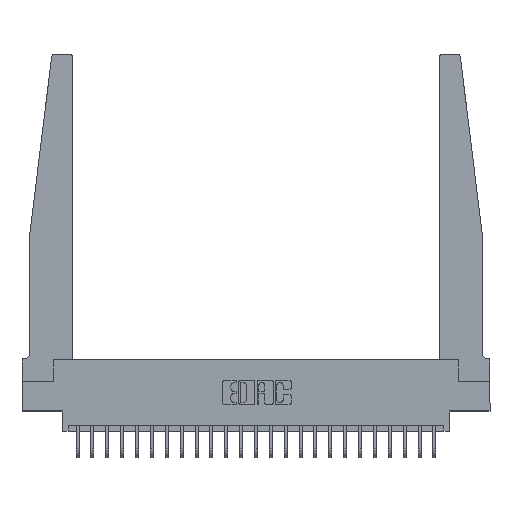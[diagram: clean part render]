
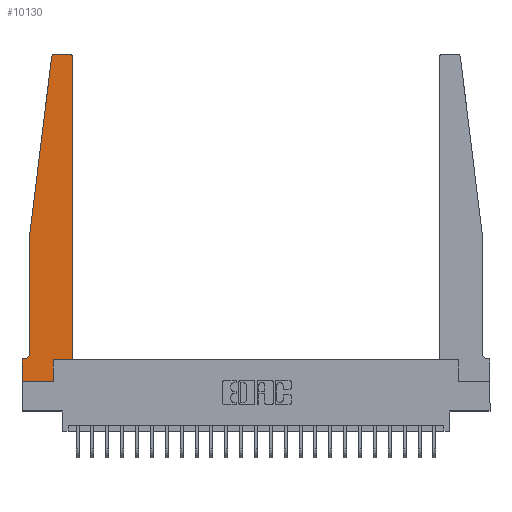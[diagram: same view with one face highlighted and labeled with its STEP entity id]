
A CAD part, top view. The second image highlights one B-rep face of the part: STEP entity #10130.
In plain terms, the highlighted planar face has unit normal (0, 0, 1).
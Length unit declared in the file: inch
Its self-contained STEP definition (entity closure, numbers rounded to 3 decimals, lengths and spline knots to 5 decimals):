
#24 = AXIS2_PLACEMENT_3D ( 'NONE', #8499, #18407, #4468 ) ;
#304 = EDGE_CURVE ( 'NONE', #21043, #7195, #3817, .T. ) ;
#314 = CARTESIAN_POINT ( 'NONE',  ( 0.2605, 0., 0.37 ) ) ;
#381 = VERTEX_POINT ( 'NONE', #2882 ) ;
#1046 = CARTESIAN_POINT ( 'NONE',  ( 0.425, 2.72, 0.37 ) ) ;
#1355 = AXIS2_PLACEMENT_3D ( 'NONE', #11608, #19559, #1560 ) ;
#1358 = VERTEX_POINT ( 'NONE', #22112 ) ;
#1452 = CARTESIAN_POINT ( 'NONE',  ( 0.24675, 2.72367, 0.37 ) ) ;
#1560 = DIRECTION ( 'NONE',  ( 1., 0., 0. ) ) ;
#1747 = ORIENTED_EDGE ( 'NONE', *, *, #25150, .T. ) ;
#1870 = CARTESIAN_POINT ( 'NONE',  ( 0., 0., 0.37 ) ) ;
#2882 = CARTESIAN_POINT ( 'NONE',  ( 0.065, 0.2375, 0.37 ) ) ;
#2939 = VECTOR ( 'NONE', #24026, 39.37008 ) ;
#3020 = CARTESIAN_POINT ( 'NONE',  ( 0.015, 0.1875, 0.37 ) ) ;
#3391 = CARTESIAN_POINT ( 'NONE',  ( 0., 0., 0.37 ) ) ;
#3817 = LINE ( 'NONE', #11770, #8479 ) ;
#4214 = DIRECTION ( 'NONE',  ( -1., 0., 0. ) ) ;
#4343 = LINE ( 'NONE', #1870, #2939 ) ;
#4468 = DIRECTION ( 'NONE',  ( 1., 0., 0. ) ) ;
#4719 = LINE ( 'NONE', #24427, #22389 ) ;
#5228 = DIRECTION ( 'NONE',  ( 1., 0., 0. ) ) ;
#5390 = CARTESIAN_POINT ( 'NONE',  ( 0.065, 1.25, 0.37 ) ) ;
#5484 = CIRCLE ( 'NONE', #24227, 0.05 ) ;
#5533 = DIRECTION ( 'NONE',  ( 1., 0., 0. ) ) ;
#5964 = ORIENTED_EDGE ( 'NONE', *, *, #22674, .T. ) ;
#6284 = CARTESIAN_POINT ( 'NONE',  ( 0.015, 0.2375, 0.37 ) ) ;
#6424 = DIRECTION ( 'NONE',  ( 0., 0., -1. ) ) ;
#6512 = VERTEX_POINT ( 'NONE', #14844 ) ;
#6860 = ORIENTED_EDGE ( 'NONE', *, *, #19320, .T. ) ;
#6915 = CARTESIAN_POINT ( 'NONE',  ( 0.425, 0.18, 0.37 ) ) ;
#7162 = CARTESIAN_POINT ( 'NONE',  ( 0., 0.1875, 0.37 ) ) ;
#7187 = ORIENTED_EDGE ( 'NONE', *, *, #20446, .T. ) ;
#7195 = VERTEX_POINT ( 'NONE', #24451 ) ;
#7307 = PLANE ( 'NONE',  #18907 ) ;
#7450 = LINE ( 'NONE', #17235, #17343 ) ;
#8479 = VECTOR ( 'NONE', #19866, 39.37008 ) ;
#8499 = CARTESIAN_POINT ( 'NONE',  ( 0.27653, 2.72, 0.37 ) ) ;
#8793 = CARTESIAN_POINT ( 'NONE',  ( 0., 0.1875, 0.37 ) ) ;
#9030 = EDGE_CURVE ( 'NONE', #18633, #6512, #4719, .T. ) ;
#9146 = LINE ( 'NONE', #18548, #12174 ) ;
#9872 = ORIENTED_EDGE ( 'NONE', *, *, #10590, .T. ) ;
#10130 = ADVANCED_FACE ( 'NONE', ( #22931 ), #7307, .T. ) ;
#10590 = EDGE_CURVE ( 'NONE', #20733, #11001, #16542, .T. ) ;
#11001 = VERTEX_POINT ( 'NONE', #5390 ) ;
#11121 = DIRECTION ( 'NONE',  ( -1., 0., 0. ) ) ;
#11195 = DIRECTION ( 'NONE',  ( -0.122, -0.992, 0. ) ) ;
#11608 = CARTESIAN_POINT ( 'NONE',  ( 0.395, 2.72, 0.37 ) ) ;
#11770 = CARTESIAN_POINT ( 'NONE',  ( 0.2605, 0.18, 0.37 ) ) ;
#12112 = DIRECTION ( 'NONE',  ( 1., 0., 0. ) ) ;
#12174 = VECTOR ( 'NONE', #16723, 39.37008 ) ;
#12342 = VERTEX_POINT ( 'NONE', #8793 ) ;
#12706 = EDGE_CURVE ( 'NONE', #22793, #12342, #7450, .T. ) ;
#12776 = VECTOR ( 'NONE', #11195, 39.37008 ) ;
#12779 = LINE ( 'NONE', #6915, #15150 ) ;
#13474 = CARTESIAN_POINT ( 'NONE',  ( 0.425, 0.18, 0.37 ) ) ;
#13530 = VERTEX_POINT ( 'NONE', #1046 ) ;
#14291 = ORIENTED_EDGE ( 'NONE', *, *, #304, .T. ) ;
#14844 = CARTESIAN_POINT ( 'NONE',  ( 0.27653, 2.75, 0.37 ) ) ;
#15080 = CARTESIAN_POINT ( 'NONE',  ( 0.065, 1.25, 0.37 ) ) ;
#15128 = VECTOR ( 'NONE', #5533, 39.37008 ) ;
#15150 = VECTOR ( 'NONE', #18529, 39.37008 ) ;
#15222 = ORIENTED_EDGE ( 'NONE', *, *, #9030, .T. ) ;
#16318 = EDGE_LOOP ( 'NONE', ( #15222, #17565, #9872, #5964, #22297, #25455, #7187, #18895, #14291, #1747, #6860, #19409 ) ) ;
#16542 = LINE ( 'NONE', #15080, #12776 ) ;
#16723 = DIRECTION ( 'NONE',  ( 0., -1., 0. ) ) ;
#16824 = DIRECTION ( 'NONE',  ( 0., 0., 1. ) ) ;
#17220 = VECTOR ( 'NONE', #12112, 39.37008 ) ;
#17235 = CARTESIAN_POINT ( 'NONE',  ( 0.065, 0.1875, 0.37 ) ) ;
#17343 = VECTOR ( 'NONE', #23332, 39.37008 ) ;
#17565 = ORIENTED_EDGE ( 'NONE', *, *, #19516, .T. ) ;
#18407 = DIRECTION ( 'NONE',  ( 0., 0., 1. ) ) ;
#18529 = DIRECTION ( 'NONE',  ( 0., 1., 0. ) ) ;
#18548 = CARTESIAN_POINT ( 'NONE',  ( 0.065, 1.25, 0.37 ) ) ;
#18633 = VERTEX_POINT ( 'NONE', #19411 ) ;
#18895 = ORIENTED_EDGE ( 'NONE', *, *, #24547, .T. ) ;
#18907 = AXIS2_PLACEMENT_3D ( 'NONE', #7162, #16824, #5228 ) ;
#19320 = EDGE_CURVE ( 'NONE', #1358, #13530, #12779, .T. ) ;
#19409 = ORIENTED_EDGE ( 'NONE', *, *, #24499, .T. ) ;
#19411 = CARTESIAN_POINT ( 'NONE',  ( 0.395, 2.75, 0.37 ) ) ;
#19516 = EDGE_CURVE ( 'NONE', #6512, #20733, #21661, .T. ) ;
#19559 = DIRECTION ( 'NONE',  ( 0., 0., 1. ) ) ;
#19738 = LINE ( 'NONE', #13474, #15128 ) ;
#19866 = DIRECTION ( 'NONE',  ( 0., 1., 0. ) ) ;
#20446 = EDGE_CURVE ( 'NONE', #12342, #22666, #4343, .T. ) ;
#20733 = VERTEX_POINT ( 'NONE', #1452 ) ;
#21043 = VERTEX_POINT ( 'NONE', #314 ) ;
#21102 = EDGE_CURVE ( 'NONE', #381, #22793, #5484, .T. ) ;
#21249 = LINE ( 'NONE', #3391, #17220 ) ;
#21661 = CIRCLE ( 'NONE', #24, 0.03 ) ;
#22112 = CARTESIAN_POINT ( 'NONE',  ( 0.425, 0.18, 0.37 ) ) ;
#22297 = ORIENTED_EDGE ( 'NONE', *, *, #21102, .T. ) ;
#22389 = VECTOR ( 'NONE', #11121, 39.37008 ) ;
#22666 = VERTEX_POINT ( 'NONE', #22700 ) ;
#22674 = EDGE_CURVE ( 'NONE', #11001, #381, #9146, .T. ) ;
#22700 = CARTESIAN_POINT ( 'NONE',  ( 0., 0., 0.37 ) ) ;
#22793 = VERTEX_POINT ( 'NONE', #3020 ) ;
#22931 = FACE_OUTER_BOUND ( 'NONE', #16318, .T. ) ;
#23332 = DIRECTION ( 'NONE',  ( -1., 0., 0. ) ) ;
#24026 = DIRECTION ( 'NONE',  ( 0., -1., 0. ) ) ;
#24227 = AXIS2_PLACEMENT_3D ( 'NONE', #6284, #6424, #4214 ) ;
#24427 = CARTESIAN_POINT ( 'NONE',  ( 0.25, 2.75, 0.37 ) ) ;
#24451 = CARTESIAN_POINT ( 'NONE',  ( 0.2605, 0.18, 0.37 ) ) ;
#24499 = EDGE_CURVE ( 'NONE', #13530, #18633, #25114, .T. ) ;
#24547 = EDGE_CURVE ( 'NONE', #22666, #21043, #21249, .T. ) ;
#25114 = CIRCLE ( 'NONE', #1355, 0.03 ) ;
#25150 = EDGE_CURVE ( 'NONE', #7195, #1358, #19738, .T. ) ;
#25455 = ORIENTED_EDGE ( 'NONE', *, *, #12706, .T. ) ;
